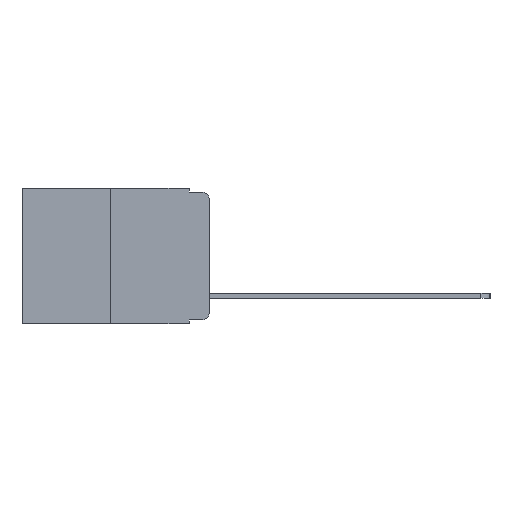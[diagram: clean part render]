
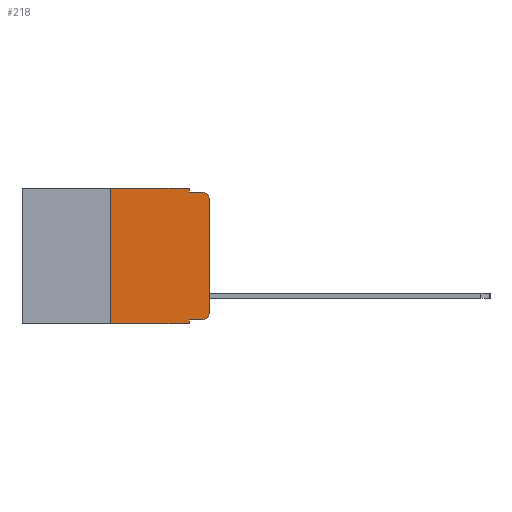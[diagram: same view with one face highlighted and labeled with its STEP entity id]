
A CAD part, left-side view. The second image highlights one B-rep face of the part: STEP entity #218.
In plain terms, the highlighted planar face has unit normal (-1, 0, 0).
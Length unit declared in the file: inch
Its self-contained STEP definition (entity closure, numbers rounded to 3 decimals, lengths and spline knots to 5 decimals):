
#60 = AXIS2_PLACEMENT_3D ( 'NONE', #1144, #13474, #3094 ) ;
#63 = LINE ( 'NONE', #12231, #13687 ) ;
#113 = VECTOR ( 'NONE', #21289, 39.37008 ) ;
#218 = ADVANCED_FACE ( 'NONE', ( #19387 ), #17400, .F. ) ;
#716 = LINE ( 'NONE', #18080, #113 ) ;
#1111 = CARTESIAN_POINT ( 'NONE',  ( 0., 0.051, 0. ) ) ;
#1144 = CARTESIAN_POINT ( 'NONE',  ( 0., 0.02, -0.313 ) ) ;
#1229 = VERTEX_POINT ( 'NONE', #3348 ) ;
#1258 = DIRECTION ( 'NONE',  ( 0., 0., 1. ) ) ;
#1495 = CARTESIAN_POINT ( 'NONE',  ( 0., 0.02, -0.03 ) ) ;
#1578 = EDGE_LOOP ( 'NONE', ( #3705, #2230, #10322, #21375, #20656, #21629, #7644, #6239, #16320, #12917 ) ) ;
#2230 = ORIENTED_EDGE ( 'NONE', *, *, #3509, .T. ) ;
#2245 = EDGE_CURVE ( 'NONE', #15838, #5041, #12581, .T. ) ;
#2330 = CARTESIAN_POINT ( 'NONE',  ( 0., 0.25, 0. ) ) ;
#3028 = LINE ( 'NONE', #21190, #15721 ) ;
#3093 = CARTESIAN_POINT ( 'NONE',  ( 0., 0.051, -0.01 ) ) ;
#3095 = DIRECTION ( 'NONE',  ( 0., 0., -1. ) ) ;
#3094 = DIRECTION ( 'NONE',  ( 0., 0., -1. ) ) ;
#3348 = CARTESIAN_POINT ( 'NONE',  ( 0., 0.25, -0.343 ) ) ;
#3436 = DIRECTION ( 'NONE',  ( 0., 0., -1. ) ) ;
#3509 = EDGE_CURVE ( 'NONE', #13498, #15637, #3859, .T. ) ;
#3705 = ORIENTED_EDGE ( 'NONE', *, *, #6763, .T. ) ;
#3859 = CIRCLE ( 'NONE', #15284, 0.02 ) ;
#4236 = VERTEX_POINT ( 'NONE', #21551 ) ;
#4265 = EDGE_CURVE ( 'NONE', #4236, #7056, #18543, .T. ) ;
#4662 = CARTESIAN_POINT ( 'NONE',  ( 0., 0., -0.03 ) ) ;
#4923 = DIRECTION ( 'NONE',  ( 0., -1., 0. ) ) ;
#5011 = VERTEX_POINT ( 'NONE', #8306 ) ;
#5041 = VERTEX_POINT ( 'NONE', #1111 ) ;
#5206 = VECTOR ( 'NONE', #1258, 39.37008 ) ;
#6120 = DIRECTION ( 'NONE',  ( 0., 0., -1. ) ) ;
#6239 = ORIENTED_EDGE ( 'NONE', *, *, #4265, .F. ) ;
#6763 = EDGE_CURVE ( 'NONE', #20645, #13498, #15059, .T. ) ;
#7056 = VERTEX_POINT ( 'NONE', #21740 ) ;
#7376 = VERTEX_POINT ( 'NONE', #10727 ) ;
#7644 = ORIENTED_EDGE ( 'NONE', *, *, #11406, .T. ) ;
#8306 = CARTESIAN_POINT ( 'NONE',  ( 0., 0.051, -0.01 ) ) ;
#8663 = VECTOR ( 'NONE', #21301, 39.37008 ) ;
#9088 = CARTESIAN_POINT ( 'NONE',  ( 0., 0.02, -0.01 ) ) ;
#9796 = CARTESIAN_POINT ( 'NONE',  ( 0., 0.473, 0. ) ) ;
#10250 = CARTESIAN_POINT ( 'NONE',  ( 0., 0.25, 0. ) ) ;
#10322 = ORIENTED_EDGE ( 'NONE', *, *, #11665, .F. ) ;
#10646 = CIRCLE ( 'NONE', #60, 0.02 ) ;
#10651 = VECTOR ( 'NONE', #11269, 39.37008 ) ;
#10727 = CARTESIAN_POINT ( 'NONE',  ( 0., 0.02, -0.333 ) ) ;
#11269 = DIRECTION ( 'NONE',  ( 0., 0., 1. ) ) ;
#11406 = EDGE_CURVE ( 'NONE', #1229, #7056, #716, .T. ) ;
#11665 = EDGE_CURVE ( 'NONE', #5011, #15637, #17901, .T. ) ;
#11799 = CARTESIAN_POINT ( 'NONE',  ( 0., 0.051, 0. ) ) ;
#12231 = CARTESIAN_POINT ( 'NONE',  ( 0., 0.051, -0.333 ) ) ;
#12380 = EDGE_CURVE ( 'NONE', #4236, #7376, #63, .T. ) ;
#12581 = LINE ( 'NONE', #9796, #8663 ) ;
#12917 = ORIENTED_EDGE ( 'NONE', *, *, #16852, .T. ) ;
#13474 = DIRECTION ( 'NONE',  ( -1., 0., 0. ) ) ;
#13498 = VERTEX_POINT ( 'NONE', #4662 ) ;
#13499 = CARTESIAN_POINT ( 'NONE',  ( 0., 0.473, 0. ) ) ;
#13687 = VECTOR ( 'NONE', #13899, 39.37008 ) ;
#13773 = DIRECTION ( 'NONE',  ( -1., 0., 0. ) ) ;
#13899 = DIRECTION ( 'NONE',  ( 0., -1., 0. ) ) ;
#13911 = EDGE_CURVE ( 'NONE', #5041, #5011, #3028, .T. ) ;
#14123 = VECTOR ( 'NONE', #3095, 39.37008 ) ;
#15059 = LINE ( 'NONE', #19515, #10651 ) ;
#15284 = AXIS2_PLACEMENT_3D ( 'NONE', #1495, #13773, #3436 ) ;
#15637 = VERTEX_POINT ( 'NONE', #9088 ) ;
#15721 = VECTOR ( 'NONE', #6120, 39.37008 ) ;
#15838 = VERTEX_POINT ( 'NONE', #2330 ) ;
#16144 = EDGE_CURVE ( 'NONE', #1229, #15838, #19223, .T. ) ;
#16320 = ORIENTED_EDGE ( 'NONE', *, *, #12380, .T. ) ;
#16415 = AXIS2_PLACEMENT_3D ( 'NONE', #13499, #19882, #19526 ) ;
#16852 = EDGE_CURVE ( 'NONE', #7376, #20645, #10646, .T. ) ;
#17400 = PLANE ( 'NONE',  #16415 ) ;
#17901 = LINE ( 'NONE', #3093, #21635 ) ;
#18080 = CARTESIAN_POINT ( 'NONE',  ( 0., 0.473, -0.343 ) ) ;
#18543 = LINE ( 'NONE', #11799, #14123 ) ;
#18954 = CARTESIAN_POINT ( 'NONE',  ( 0., 0., -0.313 ) ) ;
#19223 = LINE ( 'NONE', #10250, #5206 ) ;
#19387 = FACE_OUTER_BOUND ( 'NONE', #1578, .T. ) ;
#19515 = CARTESIAN_POINT ( 'NONE',  ( 0., 0., 0. ) ) ;
#19526 = DIRECTION ( 'NONE',  ( 0., 0., -1. ) ) ;
#19882 = DIRECTION ( 'NONE',  ( 1., 0., 0. ) ) ;
#20645 = VERTEX_POINT ( 'NONE', #18954 ) ;
#20656 = ORIENTED_EDGE ( 'NONE', *, *, #2245, .F. ) ;
#21190 = CARTESIAN_POINT ( 'NONE',  ( 0., 0.051, 0. ) ) ;
#21289 = DIRECTION ( 'NONE',  ( 0., -1., 0. ) ) ;
#21301 = DIRECTION ( 'NONE',  ( 0., -1., 0. ) ) ;
#21375 = ORIENTED_EDGE ( 'NONE', *, *, #13911, .F. ) ;
#21551 = CARTESIAN_POINT ( 'NONE',  ( 0., 0.051, -0.333 ) ) ;
#21629 = ORIENTED_EDGE ( 'NONE', *, *, #16144, .F. ) ;
#21635 = VECTOR ( 'NONE', #4923, 39.37008 ) ;
#21740 = CARTESIAN_POINT ( 'NONE',  ( 0., 0.051, -0.343 ) ) ;
